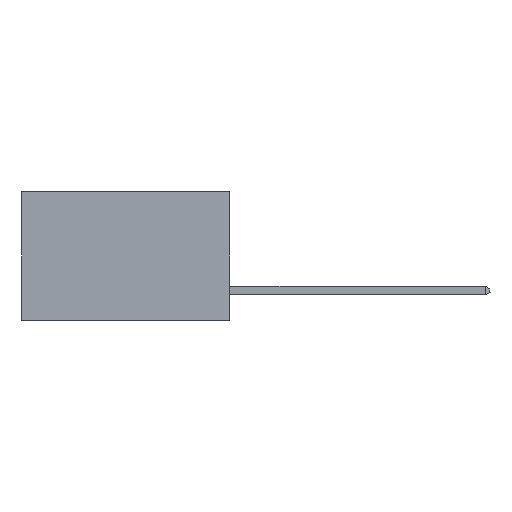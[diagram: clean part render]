
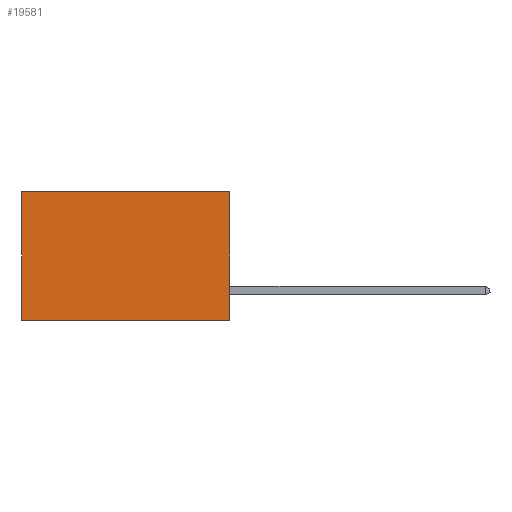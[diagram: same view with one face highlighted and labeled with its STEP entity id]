
A CAD part, left-side view. The second image highlights one B-rep face of the part: STEP entity #19581.
In plain terms, the highlighted planar face has unit normal (-1, 0, 0).
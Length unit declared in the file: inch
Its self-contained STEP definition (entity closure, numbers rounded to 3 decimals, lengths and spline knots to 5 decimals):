
#117 = EDGE_CURVE ( 'NONE', #24211, #4013, #19506, .T. ) ;
#1232 = PLANE ( 'NONE',  #25745 ) ;
#1663 = DIRECTION ( 'NONE',  ( 0., 1., 0. ) ) ;
#1881 = VERTEX_POINT ( 'NONE', #8692 ) ;
#3419 = DIRECTION ( 'NONE',  ( 0., 0., -1. ) ) ;
#3815 = EDGE_CURVE ( 'NONE', #24211, #25373, #18222, .T. ) ;
#4013 = VERTEX_POINT ( 'NONE', #12128 ) ;
#4203 = FACE_OUTER_BOUND ( 'NONE', #17219, .T. ) ;
#5987 = ORIENTED_EDGE ( 'NONE', *, *, #117, .T. ) ;
#7197 = EDGE_CURVE ( 'NONE', #25373, #1881, #18336, .T. ) ;
#8177 = EDGE_CURVE ( 'NONE', #4013, #1881, #21702, .T. ) ;
#8692 = CARTESIAN_POINT ( 'NONE',  ( 0.298, 0.6, -0.37 ) ) ;
#10280 = CARTESIAN_POINT ( 'NONE',  ( 0.298, 0., -0.37 ) ) ;
#10559 = CARTESIAN_POINT ( 'NONE',  ( 0.298, 0.6, 0. ) ) ;
#11035 = ORIENTED_EDGE ( 'NONE', *, *, #8177, .T. ) ;
#12128 = CARTESIAN_POINT ( 'NONE',  ( 0.298, 0.6, 0. ) ) ;
#14347 = ORIENTED_EDGE ( 'NONE', *, *, #7197, .F. ) ;
#15247 = VECTOR ( 'NONE', #1663, 39.37008 ) ;
#15558 = VECTOR ( 'NONE', #25775, 39.37008 ) ;
#16057 = VECTOR ( 'NONE', #20914, 39.37008 ) ;
#16506 = DIRECTION ( 'NONE',  ( 1., 0., 0. ) ) ;
#17219 = EDGE_LOOP ( 'NONE', ( #11035, #14347, #19963, #5987 ) ) ;
#17843 = CARTESIAN_POINT ( 'NONE',  ( 0.298, 0., -0.37 ) ) ;
#17867 = CARTESIAN_POINT ( 'NONE',  ( 0.298, 0., 0. ) ) ;
#18222 = LINE ( 'NONE', #17867, #21288 ) ;
#18336 = LINE ( 'NONE', #10280, #15247 ) ;
#19506 = LINE ( 'NONE', #21420, #16057 ) ;
#19581 = ADVANCED_FACE ( 'NONE', ( #4203 ), #1232, .F. ) ;
#19963 = ORIENTED_EDGE ( 'NONE', *, *, #3815, .F. ) ;
#19976 = DIRECTION ( 'NONE',  ( 0., 0., -1. ) ) ;
#20914 = DIRECTION ( 'NONE',  ( 0., 1., 0. ) ) ;
#21288 = VECTOR ( 'NONE', #19976, 39.37008 ) ;
#21420 = CARTESIAN_POINT ( 'NONE',  ( 0.298, 0., 0. ) ) ;
#21702 = LINE ( 'NONE', #10559, #15558 ) ;
#24211 = VERTEX_POINT ( 'NONE', #27748 ) ;
#25099 = CARTESIAN_POINT ( 'NONE',  ( 0.298, 0., 0. ) ) ;
#25373 = VERTEX_POINT ( 'NONE', #17843 ) ;
#25745 = AXIS2_PLACEMENT_3D ( 'NONE', #25099, #16506, #3419 ) ;
#25775 = DIRECTION ( 'NONE',  ( 0., 0., -1. ) ) ;
#27748 = CARTESIAN_POINT ( 'NONE',  ( 0.298, 0., 0. ) ) ;
